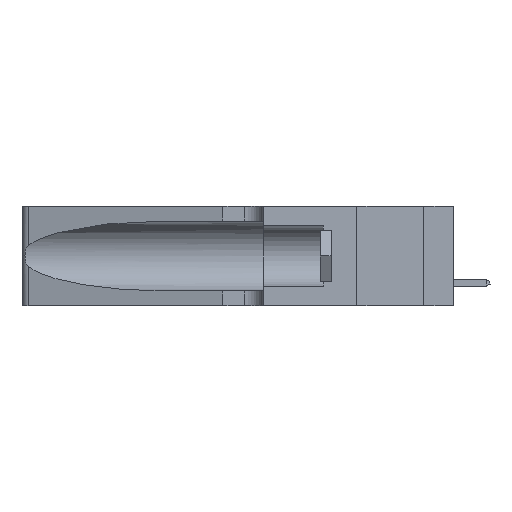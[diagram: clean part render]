
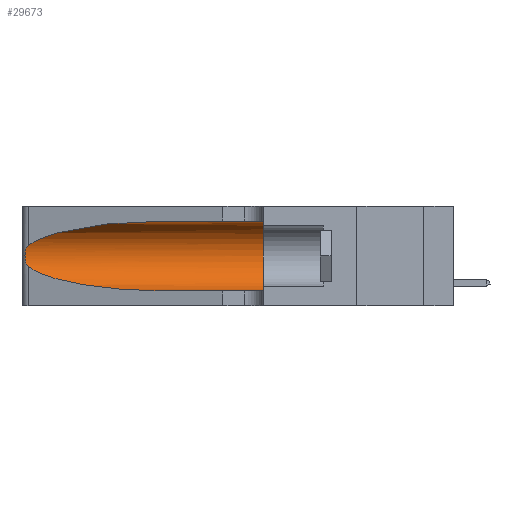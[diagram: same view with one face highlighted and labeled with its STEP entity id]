
A CAD part, left-side view. The second image highlights one B-rep face of the part: STEP entity #29673.
In plain terms, the highlighted cylindrical face has radius 3.308 mm (diameter 6.617 mm), a partial arc.
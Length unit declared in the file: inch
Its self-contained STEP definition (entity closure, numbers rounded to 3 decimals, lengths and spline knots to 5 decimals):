
#53 =( BOUNDED_CURVE ( )  B_SPLINE_CURVE ( 3, ( #41811, #21902, #21765, #8519 ),
 .UNSPECIFIED., .F., .F. ) 
 B_SPLINE_CURVE_WITH_KNOTS ( ( 4, 4 ),
 ( 3.44316, 4.71239 ),
 .UNSPECIFIED. ) 
 CURVE ( )  GEOMETRIC_REPRESENTATION_ITEM ( )  RATIONAL_B_SPLINE_CURVE ( ( 1., 0.87, 0.87, 1. ) ) 
 REPRESENTATION_ITEM ( '' )  );
#67 = EDGE_CURVE ( 'NONE', #41974, #1757, #32281, .T. ) ;
#1757 = VERTEX_POINT ( 'NONE', #10131 ) ;
#2218 = EDGE_CURVE ( 'NONE', #1757, #13687, #40462, .T. ) ;
#2696 = DIRECTION ( 'NONE',  ( 0., -1., 0. ) ) ;
#3125 = VERTEX_POINT ( 'NONE', #38311 ) ;
#3163 = ORIENTED_EDGE ( 'NONE', *, *, #36625, .T. ) ;
#3947 = ORIENTED_EDGE ( 'NONE', *, *, #17752, .T. ) ;
#4424 = CYLINDRICAL_SURFACE ( 'NONE', #11561, 0.13025 ) ;
#5879 = B_SPLINE_CURVE_WITH_KNOTS ( 'NONE', 3,
 ( #31801, #22028, #25094, #38829, #28440, #8500, #15212, #38543, #21875, #11990, #28581, #29583, #9501, #36337 ),
 .UNSPECIFIED., .F., .F.,
 ( 4, 2, 2, 2, 2, 2, 4 ),
 ( 0., 0.00027, 0.00053, 0.00107, 0.0016, 0.00187, 0.00214 ),
 .UNSPECIFIED. ) ;
#8494 = ORIENTED_EDGE ( 'NONE', *, *, #2218, .F. ) ;
#8500 = CARTESIAN_POINT ( 'NONE',  ( 0.26018, 1.23835, 0.19895 ) ) ;
#8519 = CARTESIAN_POINT ( 'NONE',  ( 0.1305, 0.72297, 0.05475 ) ) ;
#9435 = CARTESIAN_POINT ( 'NONE',  ( 0.1305, 0.72297, 0.31525 ) ) ;
#9501 = CARTESIAN_POINT ( 'NONE',  ( 0.25555, 1.22993, 0.14849 ) ) ;
#10131 = CARTESIAN_POINT ( 'NONE',  ( 0.1305, 0.35, 0.31525 ) ) ;
#10275 = DIRECTION ( 'NONE',  ( 0., -1., 0. ) ) ;
#11561 = AXIS2_PLACEMENT_3D ( 'NONE', #29779, #10275, #23075 ) ;
#11990 = CARTESIAN_POINT ( 'NONE',  ( 0.25856, 1.23593, 0.16098 ) ) ;
#13125 = CARTESIAN_POINT ( 'NONE',  ( 0.25487, 1.22718, 0.22369 ) ) ;
#13687 = VERTEX_POINT ( 'NONE', #38167 ) ;
#13744 = CARTESIAN_POINT ( 'NONE',  ( 0.2373, 1.15595, 0.28018 ) ) ;
#15212 = CARTESIAN_POINT ( 'NONE',  ( 0.26075, 1.23896, 0.19203 ) ) ;
#16409 = FACE_OUTER_BOUND ( 'NONE', #34556, .T. ) ;
#16461 = ORIENTED_EDGE ( 'NONE', *, *, #33538, .T. ) ;
#16676 = CARTESIAN_POINT ( 'NONE',  ( 0.1305, 1.61858, 0.05475 ) ) ;
#17752 = EDGE_CURVE ( 'NONE', #41974, #3125, #30414, .T. ) ;
#18100 = CARTESIAN_POINT ( 'NONE',  ( 0.18966, 0.96281, 0.31525 ) ) ;
#18151 = AXIS2_PLACEMENT_3D ( 'NONE', #29582, #42760, #36336 ) ;
#20263 = ORIENTED_EDGE ( 'NONE', *, *, #30131, .T. ) ;
#21765 = CARTESIAN_POINT ( 'NONE',  ( 0.18966, 0.96281, 0.05475 ) ) ;
#21875 = CARTESIAN_POINT ( 'NONE',  ( 0.26017, 1.23833, 0.17102 ) ) ;
#21902 = CARTESIAN_POINT ( 'NONE',  ( 0.2373, 1.15595, 0.08982 ) ) ;
#22028 = CARTESIAN_POINT ( 'NONE',  ( 0.25555, 1.22994, 0.2215 ) ) ;
#23075 = DIRECTION ( 'NONE',  ( 0., 0., -1. ) ) ;
#25094 = CARTESIAN_POINT ( 'NONE',  ( 0.25639, 1.23184, 0.21858 ) ) ;
#25411 = LINE ( 'NONE', #16676, #42163 ) ;
#27470 = CARTESIAN_POINT ( 'NONE',  ( 0.1305, 0.72297, 0.05475 ) ) ;
#28440 = CARTESIAN_POINT ( 'NONE',  ( 0.25854, 1.2359, 0.20912 ) ) ;
#28581 = CARTESIAN_POINT ( 'NONE',  ( 0.25789, 1.23486, 0.15765 ) ) ;
#28746 = CARTESIAN_POINT ( 'NONE',  ( 0.1305, 1.61858, 0.31525 ) ) ;
#29582 = CARTESIAN_POINT ( 'NONE',  ( 0.1305, 0.35, 0.185 ) ) ;
#29583 = CARTESIAN_POINT ( 'NONE',  ( 0.25639, 1.23186, 0.15144 ) ) ;
#29627 = DIRECTION ( 'NONE',  ( 0., -1., 0. ) ) ;
#29673 = ADVANCED_FACE ( 'NONE', ( #16409 ), #4424, .F. ) ;
#29779 = CARTESIAN_POINT ( 'NONE',  ( 0.1305, 1.61858, 0.185 ) ) ;
#30131 = EDGE_CURVE ( 'NONE', #3125, #37487, #5879, .T. ) ;
#30414 =( BOUNDED_CURVE ( )  B_SPLINE_CURVE ( 3, ( #38096, #18100, #13744, #13125 ),
 .UNSPECIFIED., .F., .T. ) 
 B_SPLINE_CURVE_WITH_KNOTS ( ( 4, 4 ),
 ( 1.5708, 2.84003 ),
 .UNSPECIFIED. ) 
 CURVE ( )  GEOMETRIC_REPRESENTATION_ITEM ( )  RATIONAL_B_SPLINE_CURVE ( ( 1., 0.87, 0.87, 1. ) ) 
 REPRESENTATION_ITEM ( '' )  );
#31233 = CARTESIAN_POINT ( 'NONE',  ( 0.25487, 1.22718, 0.14631 ) ) ;
#31765 = VERTEX_POINT ( 'NONE', #27470 ) ;
#31801 = CARTESIAN_POINT ( 'NONE',  ( 0.25487, 1.22718, 0.22369 ) ) ;
#32281 = LINE ( 'NONE', #28746, #36518 ) ;
#33538 = EDGE_CURVE ( 'NONE', #31765, #13687, #25411, .T. ) ;
#34556 = EDGE_LOOP ( 'NONE', ( #3947, #20263, #3163, #16461, #8494, #36782 ) ) ;
#36336 = DIRECTION ( 'NONE',  ( 0., 0., 1. ) ) ;
#36337 = CARTESIAN_POINT ( 'NONE',  ( 0.25487, 1.22718, 0.14631 ) ) ;
#36518 = VECTOR ( 'NONE', #2696, 39.37008 ) ;
#36625 = EDGE_CURVE ( 'NONE', #37487, #31765, #53, .T. ) ;
#36782 = ORIENTED_EDGE ( 'NONE', *, *, #67, .F. ) ;
#37487 = VERTEX_POINT ( 'NONE', #31233 ) ;
#38096 = CARTESIAN_POINT ( 'NONE',  ( 0.1305, 0.72297, 0.31525 ) ) ;
#38167 = CARTESIAN_POINT ( 'NONE',  ( 0.1305, 0.35, 0.05475 ) ) ;
#38311 = CARTESIAN_POINT ( 'NONE',  ( 0.25487, 1.22718, 0.22369 ) ) ;
#38543 = CARTESIAN_POINT ( 'NONE',  ( 0.26075, 1.23896, 0.178 ) ) ;
#38829 = CARTESIAN_POINT ( 'NONE',  ( 0.25787, 1.23484, 0.2124 ) ) ;
#40462 = CIRCLE ( 'NONE', #18151, 0.13025 ) ;
#41811 = CARTESIAN_POINT ( 'NONE',  ( 0.25487, 1.22718, 0.14631 ) ) ;
#41974 = VERTEX_POINT ( 'NONE', #9435 ) ;
#42163 = VECTOR ( 'NONE', #29627, 39.37008 ) ;
#42760 = DIRECTION ( 'NONE',  ( 0., 1., 0. ) ) ;
